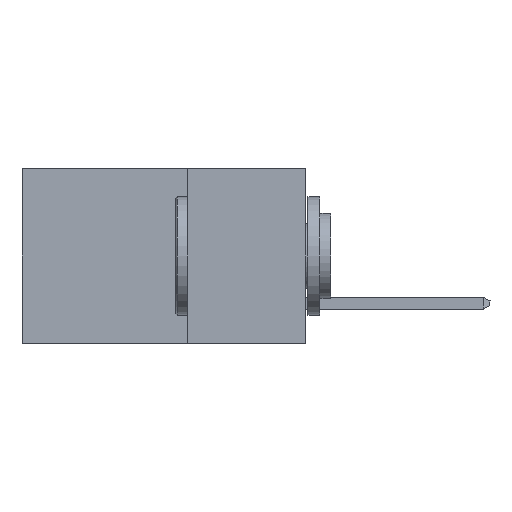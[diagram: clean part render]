
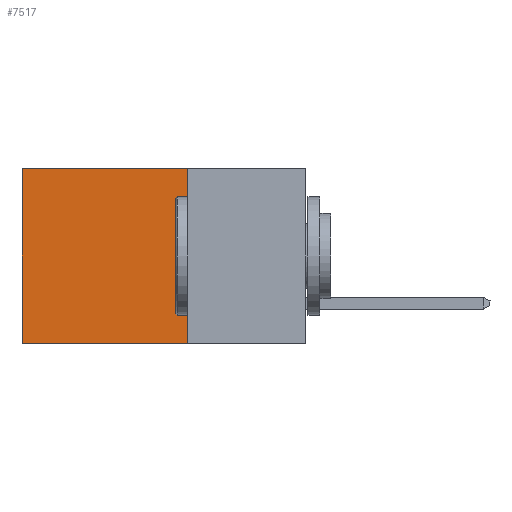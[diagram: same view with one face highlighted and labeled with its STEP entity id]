
A CAD part, left-side view. The second image highlights one B-rep face of the part: STEP entity #7517.
In plain terms, the highlighted planar face has unit normal (-1, 0, 0).
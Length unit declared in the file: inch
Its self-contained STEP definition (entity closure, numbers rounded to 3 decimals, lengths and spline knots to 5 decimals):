
#1793 = ORIENTED_EDGE ( 'NONE', *, *, #5234, .T. ) ;
#2975 = EDGE_CURVE ( 'NONE', #12254, #10607, #17094, .T. ) ;
#3462 = DIRECTION ( 'NONE',  ( 0., 0., -1. ) ) ;
#4605 = EDGE_CURVE ( 'NONE', #16624, #8966, #15758, .T. ) ;
#4924 = CARTESIAN_POINT ( 'NONE',  ( 0.298, 0.25, 0. ) ) ;
#5234 = EDGE_CURVE ( 'NONE', #8966, #10607, #15467, .T. ) ;
#5635 = CARTESIAN_POINT ( 'NONE',  ( 0.298, 0.6, 0. ) ) ;
#7212 = VECTOR ( 'NONE', #8231, 39.37008 ) ;
#7517 = ADVANCED_FACE ( 'NONE', ( #8285 ), #13109, .F. ) ;
#7777 = EDGE_CURVE ( 'NONE', #16624, #12254, #20078, .T. ) ;
#8096 = DIRECTION ( 'NONE',  ( 0., 1., 0. ) ) ;
#8125 = CARTESIAN_POINT ( 'NONE',  ( 0.298, 0.25, 0. ) ) ;
#8197 = DIRECTION ( 'NONE',  ( 1., 0., 0. ) ) ;
#8231 = DIRECTION ( 'NONE',  ( 0., 1., 0. ) ) ;
#8285 = FACE_OUTER_BOUND ( 'NONE', #10357, .T. ) ;
#8966 = VERTEX_POINT ( 'NONE', #5635 ) ;
#10305 = ORIENTED_EDGE ( 'NONE', *, *, #7777, .F. ) ;
#10357 = EDGE_LOOP ( 'NONE', ( #1793, #13103, #10305, #10444 ) ) ;
#10444 = ORIENTED_EDGE ( 'NONE', *, *, #4605, .T. ) ;
#10607 = VERTEX_POINT ( 'NONE', #17356 ) ;
#11089 = CARTESIAN_POINT ( 'NONE',  ( 0.298, 0.25, 0. ) ) ;
#11507 = VECTOR ( 'NONE', #12731, 39.37008 ) ;
#12254 = VERTEX_POINT ( 'NONE', #20156 ) ;
#12731 = DIRECTION ( 'NONE',  ( 0., 0., -1. ) ) ;
#12792 = CARTESIAN_POINT ( 'NONE',  ( 0.298, 0.25, 0. ) ) ;
#12877 = CARTESIAN_POINT ( 'NONE',  ( 0.298, 0.25, -0.37 ) ) ;
#13103 = ORIENTED_EDGE ( 'NONE', *, *, #2975, .F. ) ;
#13109 = PLANE ( 'NONE',  #14316 ) ;
#13613 = CARTESIAN_POINT ( 'NONE',  ( 0.298, 0.6, 0. ) ) ;
#14316 = AXIS2_PLACEMENT_3D ( 'NONE', #8125, #8197, #3462 ) ;
#15208 = DIRECTION ( 'NONE',  ( 0., 0., -1. ) ) ;
#15467 = LINE ( 'NONE', #13613, #19779 ) ;
#15758 = LINE ( 'NONE', #12792, #7212 ) ;
#16624 = VERTEX_POINT ( 'NONE', #4924 ) ;
#17094 = LINE ( 'NONE', #12877, #18633 ) ;
#17356 = CARTESIAN_POINT ( 'NONE',  ( 0.298, 0.6, -0.37 ) ) ;
#18633 = VECTOR ( 'NONE', #8096, 39.37008 ) ;
#19779 = VECTOR ( 'NONE', #15208, 39.37008 ) ;
#20078 = LINE ( 'NONE', #11089, #11507 ) ;
#20156 = CARTESIAN_POINT ( 'NONE',  ( 0.298, 0.25, -0.37 ) ) ;
